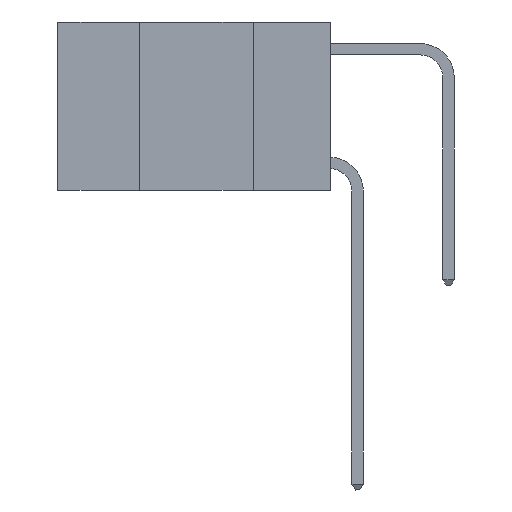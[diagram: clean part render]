
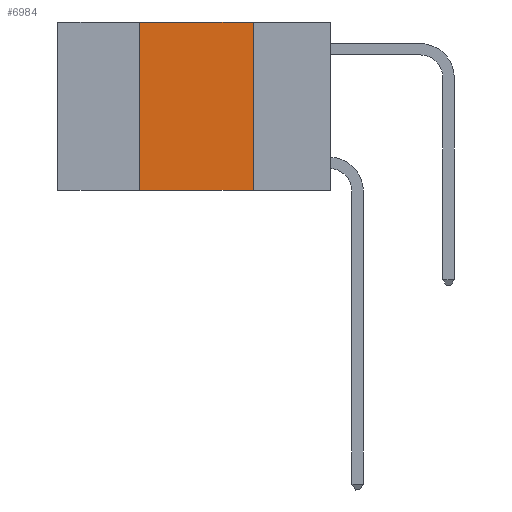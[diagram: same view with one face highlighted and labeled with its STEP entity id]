
A CAD part, left-side view. The second image highlights one B-rep face of the part: STEP entity #6984.
In plain terms, the highlighted planar face has unit normal (-1, 0, 0).
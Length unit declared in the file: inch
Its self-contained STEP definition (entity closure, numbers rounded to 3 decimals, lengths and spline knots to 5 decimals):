
#307 = CARTESIAN_POINT ( 'NONE',  ( 0., 0.42, -0.37 ) ) ;
#480 = ORIENTED_EDGE ( 'NONE', *, *, #11537, .F. ) ;
#1011 = CARTESIAN_POINT ( 'NONE',  ( 0., 0.6, 0. ) ) ;
#1442 = EDGE_CURVE ( 'NONE', #10826, #7484, #8535, .T. ) ;
#1506 = CARTESIAN_POINT ( 'NONE',  ( 0., 0.17, 0. ) ) ;
#1795 = VECTOR ( 'NONE', #6744, 39.37008 ) ;
#1974 = CARTESIAN_POINT ( 'NONE',  ( 0., 0.17, -0.37 ) ) ;
#2189 = FACE_OUTER_BOUND ( 'NONE', #10430, .T. ) ;
#3502 = CARTESIAN_POINT ( 'NONE',  ( 0., 0.6, 0. ) ) ;
#3735 = CARTESIAN_POINT ( 'NONE',  ( 0., 0.42, 0. ) ) ;
#3998 = VERTEX_POINT ( 'NONE', #12575 ) ;
#5252 = VECTOR ( 'NONE', #13163, 39.37008 ) ;
#6744 = DIRECTION ( 'NONE',  ( 0., -1., 0. ) ) ;
#6984 = ADVANCED_FACE ( 'NONE', ( #2189 ), #13770, .F. ) ;
#7214 = DIRECTION ( 'NONE',  ( 0., -1., 0. ) ) ;
#7263 = VECTOR ( 'NONE', #7214, 39.37008 ) ;
#7297 = LINE ( 'NONE', #3735, #5252 ) ;
#7301 = DIRECTION ( 'NONE',  ( 0., 0., -1. ) ) ;
#7484 = VERTEX_POINT ( 'NONE', #1974 ) ;
#8131 = LINE ( 'NONE', #1011, #1795 ) ;
#8535 = LINE ( 'NONE', #9460, #10010 ) ;
#9460 = CARTESIAN_POINT ( 'NONE',  ( 0., 0.17, 0. ) ) ;
#9590 = LINE ( 'NONE', #11839, #7263 ) ;
#10010 = VECTOR ( 'NONE', #7301, 39.37008 ) ;
#10430 = EDGE_LOOP ( 'NONE', ( #13535, #480, #14972, #12142 ) ) ;
#10826 = VERTEX_POINT ( 'NONE', #1506 ) ;
#11239 = EDGE_CURVE ( 'NONE', #11749, #3998, #7297, .T. ) ;
#11537 = EDGE_CURVE ( 'NONE', #3998, #10826, #8131, .T. ) ;
#11749 = VERTEX_POINT ( 'NONE', #307 ) ;
#11839 = CARTESIAN_POINT ( 'NONE',  ( 0., 0.6, -0.37 ) ) ;
#12142 = ORIENTED_EDGE ( 'NONE', *, *, #13034, .T. ) ;
#12575 = CARTESIAN_POINT ( 'NONE',  ( 0., 0.42, 0. ) ) ;
#12619 = DIRECTION ( 'NONE',  ( 0., 0., -1. ) ) ;
#12767 = DIRECTION ( 'NONE',  ( 1., 0., 0. ) ) ;
#13034 = EDGE_CURVE ( 'NONE', #11749, #7484, #9590, .T. ) ;
#13163 = DIRECTION ( 'NONE',  ( 0., 0., 1. ) ) ;
#13535 = ORIENTED_EDGE ( 'NONE', *, *, #1442, .F. ) ;
#13770 = PLANE ( 'NONE',  #14727 ) ;
#14727 = AXIS2_PLACEMENT_3D ( 'NONE', #3502, #12767, #12619 ) ;
#14972 = ORIENTED_EDGE ( 'NONE', *, *, #11239, .F. ) ;
